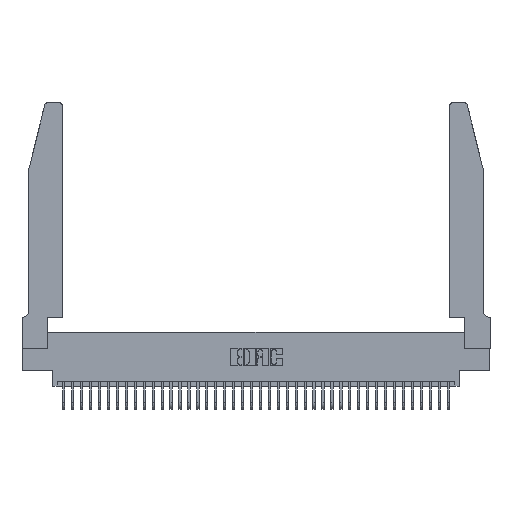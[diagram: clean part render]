
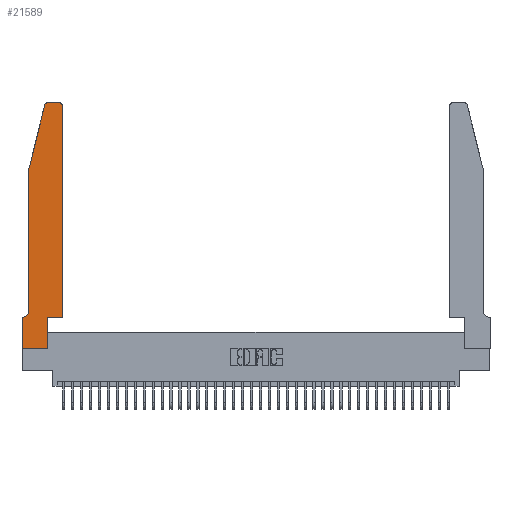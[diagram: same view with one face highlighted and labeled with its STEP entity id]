
A CAD part, top view. The second image highlights one B-rep face of the part: STEP entity #21589.
In plain terms, the highlighted planar face has unit normal (0, 0, 1).
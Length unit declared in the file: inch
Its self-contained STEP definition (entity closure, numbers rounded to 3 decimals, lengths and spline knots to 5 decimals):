
#1459 = CARTESIAN_POINT ( 'NONE',  ( 0., 0., 0.37 ) ) ;
#1965 = CARTESIAN_POINT ( 'NONE',  ( 0.0055, 0.35, 0.37 ) ) ;
#2381 = CARTESIAN_POINT ( 'NONE',  ( 0., 0.35, 0.37 ) ) ;
#2481 = DIRECTION ( 'NONE',  ( -0.239, -0.971, 0. ) ) ;
#3140 = CARTESIAN_POINT ( 'NONE',  ( 0.284, 2.75, 0.37 ) ) ;
#5227 = ORIENTED_EDGE ( 'NONE', *, *, #11504, .T. ) ;
#5367 = DIRECTION ( 'NONE',  ( 0., 0., 1. ) ) ;
#5450 = LINE ( 'NONE', #31471, #20118 ) ;
#5509 = ORIENTED_EDGE ( 'NONE', *, *, #18436, .T. ) ;
#5812 = DIRECTION ( 'NONE',  ( 0., 0., 1. ) ) ;
#5855 = CARTESIAN_POINT ( 'NONE',  ( 0., 0., 0.37 ) ) ;
#6462 = DIRECTION ( 'NONE',  ( 0., 1., 0. ) ) ;
#6626 = LINE ( 'NONE', #14547, #29916 ) ;
#6665 = LINE ( 'NONE', #19118, #21293 ) ;
#6703 = AXIS2_PLACEMENT_3D ( 'NONE', #30872, #13437, #33794 ) ;
#7103 = CARTESIAN_POINT ( 'NONE',  ( 0.0755, 2., 0.37 ) ) ;
#7312 = VERTEX_POINT ( 'NONE', #37110 ) ;
#8084 = VERTEX_POINT ( 'NONE', #15013 ) ;
#8226 = DIRECTION ( 'NONE',  ( 0., 0., 1. ) ) ;
#8502 = LINE ( 'NONE', #1459, #9406 ) ;
#8667 = ORIENTED_EDGE ( 'NONE', *, *, #37821, .T. ) ;
#9017 = FACE_OUTER_BOUND ( 'NONE', #34727, .T. ) ;
#9406 = VECTOR ( 'NONE', #21940, 39.37008 ) ;
#9695 = EDGE_CURVE ( 'NONE', #30588, #23332, #13879, .T. ) ;
#9913 = EDGE_CURVE ( 'NONE', #11285, #26185, #28885, .T. ) ;
#10344 = DIRECTION ( 'NONE',  ( 0., 1., 0. ) ) ;
#11018 = ORIENTED_EDGE ( 'NONE', *, *, #9913, .T. ) ;
#11195 = LINE ( 'NONE', #32092, #34470 ) ;
#11285 = VERTEX_POINT ( 'NONE', #3140 ) ;
#11504 = EDGE_CURVE ( 'NONE', #26291, #18682, #26485, .T. ) ;
#11541 = CARTESIAN_POINT ( 'NONE',  ( 0.4505, 0.35, 0.37 ) ) ;
#11594 = AXIS2_PLACEMENT_3D ( 'NONE', #23298, #5812, #26229 ) ;
#12608 = EDGE_CURVE ( 'NONE', #8084, #15932, #36383, .T. ) ;
#12965 = CARTESIAN_POINT ( 'NONE',  ( 0., 0., 0.37 ) ) ;
#13437 = DIRECTION ( 'NONE',  ( 0., 0., -1. ) ) ;
#13879 = LINE ( 'NONE', #18127, #28456 ) ;
#14547 = CARTESIAN_POINT ( 'NONE',  ( 0.2605, 2.75, 0.37 ) ) ;
#14705 = DIRECTION ( 'NONE',  ( -1., 0., 0. ) ) ;
#15013 = CARTESIAN_POINT ( 'NONE',  ( 0.4505, 2.72, 0.37 ) ) ;
#15417 = EDGE_CURVE ( 'NONE', #26185, #26291, #5450, .T. ) ;
#15437 = ORIENTED_EDGE ( 'NONE', *, *, #26882, .T. ) ;
#15932 = VERTEX_POINT ( 'NONE', #16684 ) ;
#16094 = VERTEX_POINT ( 'NONE', #11541 ) ;
#16684 = CARTESIAN_POINT ( 'NONE',  ( 0.4205, 2.75, 0.37 ) ) ;
#17111 = ORIENTED_EDGE ( 'NONE', *, *, #15417, .T. ) ;
#17134 = CARTESIAN_POINT ( 'NONE',  ( 0.0755, 0.42, 0.37 ) ) ;
#17183 = VECTOR ( 'NONE', #10344, 39.37008 ) ;
#17211 = LINE ( 'NONE', #12965, #31764 ) ;
#17447 = AXIS2_PLACEMENT_3D ( 'NONE', #25705, #8226, #28652 ) ;
#18127 = CARTESIAN_POINT ( 'NONE',  ( 0.2865, 0.35, 0.37 ) ) ;
#18436 = EDGE_CURVE ( 'NONE', #16094, #8084, #34482, .T. ) ;
#18682 = VERTEX_POINT ( 'NONE', #17134 ) ;
#19118 = CARTESIAN_POINT ( 'NONE',  ( 0.4505, 0.35, 0.37 ) ) ;
#19243 = ORIENTED_EDGE ( 'NONE', *, *, #12608, .T. ) ;
#19270 = ORIENTED_EDGE ( 'NONE', *, *, #27615, .T. ) ;
#19660 = VECTOR ( 'NONE', #27546, 39.37008 ) ;
#20118 = VECTOR ( 'NONE', #2481, 39.37008 ) ;
#21293 = VECTOR ( 'NONE', #36501, 39.37008 ) ;
#21589 = ADVANCED_FACE ( 'NONE', ( #9017 ), #37329, .T. ) ;
#21771 = DIRECTION ( 'NONE',  ( 1., 0., 0. ) ) ;
#21940 = DIRECTION ( 'NONE',  ( 0., -1., 0. ) ) ;
#22009 = VERTEX_POINT ( 'NONE', #1965 ) ;
#23298 = CARTESIAN_POINT ( 'NONE',  ( 0.4205, 2.72, 0.37 ) ) ;
#23332 = VERTEX_POINT ( 'NONE', #24485 ) ;
#24485 = CARTESIAN_POINT ( 'NONE',  ( 0.2865, 0.35, 0.37 ) ) ;
#24887 = CARTESIAN_POINT ( 'NONE',  ( 0.4505, 0.35, 0.37 ) ) ;
#25705 = CARTESIAN_POINT ( 'NONE',  ( 0.284, 2.72, 0.37 ) ) ;
#25769 = DIRECTION ( 'NONE',  ( 1., 0., 0. ) ) ;
#26185 = VERTEX_POINT ( 'NONE', #33388 ) ;
#26199 = EDGE_CURVE ( 'NONE', #7312, #36586, #8502, .T. ) ;
#26229 = DIRECTION ( 'NONE',  ( 1., 0., 0. ) ) ;
#26291 = VERTEX_POINT ( 'NONE', #36803 ) ;
#26485 = LINE ( 'NONE', #7103, #19660 ) ;
#26548 = EDGE_CURVE ( 'NONE', #22009, #7312, #11195, .T. ) ;
#26882 = EDGE_CURVE ( 'NONE', #36586, #30588, #17211, .T. ) ;
#26964 = EDGE_CURVE ( 'NONE', #23332, #16094, #6665, .T. ) ;
#27546 = DIRECTION ( 'NONE',  ( 0., -1., 0. ) ) ;
#27615 = EDGE_CURVE ( 'NONE', #18682, #22009, #29445, .T. ) ;
#27913 = ORIENTED_EDGE ( 'NONE', *, *, #26964, .T. ) ;
#28456 = VECTOR ( 'NONE', #6462, 39.37008 ) ;
#28652 = DIRECTION ( 'NONE',  ( 1., 0., 0. ) ) ;
#28781 = CARTESIAN_POINT ( 'NONE',  ( 0.2865, 0., 0.37 ) ) ;
#28885 = CIRCLE ( 'NONE', #17447, 0.03 ) ;
#29445 = CIRCLE ( 'NONE', #6703, 0.07 ) ;
#29916 = VECTOR ( 'NONE', #34873, 39.37008 ) ;
#30588 = VERTEX_POINT ( 'NONE', #28781 ) ;
#30768 = ORIENTED_EDGE ( 'NONE', *, *, #26199, .T. ) ;
#30872 = CARTESIAN_POINT ( 'NONE',  ( 0.0055, 0.42, 0.37 ) ) ;
#31471 = CARTESIAN_POINT ( 'NONE',  ( 0.0755, 2., 0.37 ) ) ;
#31764 = VECTOR ( 'NONE', #21771, 39.37008 ) ;
#32092 = CARTESIAN_POINT ( 'NONE',  ( 0.0755, 0.35, 0.37 ) ) ;
#33388 = CARTESIAN_POINT ( 'NONE',  ( 0.25487, 2.72718, 0.37 ) ) ;
#33794 = DIRECTION ( 'NONE',  ( -1., 0., 0. ) ) ;
#34470 = VECTOR ( 'NONE', #14705, 39.37008 ) ;
#34482 = LINE ( 'NONE', #24887, #17183 ) ;
#34727 = EDGE_LOOP ( 'NONE', ( #8667, #11018, #17111, #5227, #19270, #34733, #30768, #15437, #35367, #27913, #5509, #19243 ) ) ;
#34733 = ORIENTED_EDGE ( 'NONE', *, *, #26548, .T. ) ;
#34873 = DIRECTION ( 'NONE',  ( -1., 0., 0. ) ) ;
#35367 = ORIENTED_EDGE ( 'NONE', *, *, #9695, .T. ) ;
#35629 = AXIS2_PLACEMENT_3D ( 'NONE', #2381, #5367, #25769 ) ;
#36383 = CIRCLE ( 'NONE', #11594, 0.03 ) ;
#36501 = DIRECTION ( 'NONE',  ( 1., 0., 0. ) ) ;
#36586 = VERTEX_POINT ( 'NONE', #5855 ) ;
#36803 = CARTESIAN_POINT ( 'NONE',  ( 0.0755, 2., 0.37 ) ) ;
#37110 = CARTESIAN_POINT ( 'NONE',  ( 0., 0.35, 0.37 ) ) ;
#37329 = PLANE ( 'NONE',  #35629 ) ;
#37821 = EDGE_CURVE ( 'NONE', #15932, #11285, #6626, .T. ) ;
